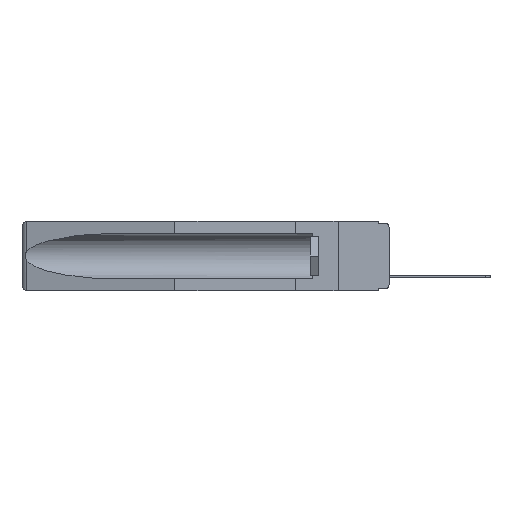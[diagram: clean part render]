
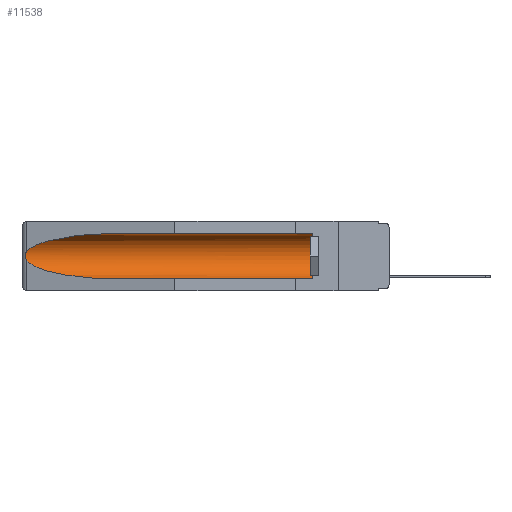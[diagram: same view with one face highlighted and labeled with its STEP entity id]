
A CAD part, left-side view. The second image highlights one B-rep face of the part: STEP entity #11538.
In plain terms, the highlighted cylindrical face has radius 2.857 mm (diameter 5.715 mm), a partial arc.
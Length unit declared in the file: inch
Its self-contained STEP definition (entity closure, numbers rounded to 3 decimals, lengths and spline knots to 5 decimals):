
#32 = CARTESIAN_POINT ( 'NONE',  ( 0.26537, 1.52718, -0.14972 ) ) ;
#301 = VECTOR ( 'NONE', #18161, 39.37008 ) ;
#348 = CARTESIAN_POINT ( 'NONE',  ( 0.155, 0.126, -0.059 ) ) ;
#428 = CARTESIAN_POINT ( 'NONE',  ( 0.26597, 1.5296, -0.19026 ) ) ;
#475 = CARTESIAN_POINT ( 'NONE',  ( 0.26537, 1.52718, -0.14972 ) ) ;
#616 = DIRECTION ( 'NONE',  ( 0., 0., 1. ) ) ;
#726 = CARTESIAN_POINT ( 'NONE',  ( 0.26537, 1.52718, -0.14972 ) ) ;
#1093 = ORIENTED_EDGE ( 'NONE', *, *, #1783, .F. ) ;
#1783 = EDGE_CURVE ( 'NONE', #4860, #5877, #4984, .T. ) ;
#1796 = ORIENTED_EDGE ( 'NONE', *, *, #17693, .T. ) ;
#2047 = CARTESIAN_POINT ( 'NONE',  ( 0.155, -0.30754, -0.1715 ) ) ;
#2898 = EDGE_CURVE ( 'NONE', #9815, #5777, #5706, .T. ) ;
#2907 = CIRCLE ( 'NONE', #16895, 0.1125 ) ;
#3389 = CARTESIAN_POINT ( 'NONE',  ( 0.155, -0.30754, -0.284 ) ) ;
#4310 = CARTESIAN_POINT ( 'NONE',  ( 0.155, 0.126, -0.1715 ) ) ;
#4643 = CARTESIAN_POINT ( 'NONE',  ( 0.155, 1.07973, -0.059 ) ) ;
#4745 = EDGE_CURVE ( 'NONE', #4860, #9815, #2907, .T. ) ;
#4860 = VERTEX_POINT ( 'NONE', #18361 ) ;
#4984 = LINE ( 'NONE', #3389, #15197 ) ;
#5153 = CARTESIAN_POINT ( 'NONE',  ( 0.26654, 1.53092, -0.15636 ) ) ;
#5706 = LINE ( 'NONE', #6013, #301 ) ;
#5777 = VERTEX_POINT ( 'NONE', #4643 ) ;
#5795 = CARTESIAN_POINT ( 'NONE',  ( 0.21114, 1.30732, -0.059 ) ) ;
#5877 = VERTEX_POINT ( 'NONE', #17292 ) ;
#6013 = CARTESIAN_POINT ( 'NONE',  ( 0.155, -0.30754, -0.059 ) ) ;
#7062 = ORIENTED_EDGE ( 'NONE', *, *, #11481, .T. ) ;
#7575 = CARTESIAN_POINT ( 'NONE',  ( 0.26537, 1.52718, -0.19328 ) ) ;
#8365 = CARTESIAN_POINT ( 'NONE',  ( 0.26537, 1.52718, -0.19328 ) ) ;
#8961 = CARTESIAN_POINT ( 'NONE',  ( 0.155, 1.07973, -0.059 ) ) ;
#9081 =( BOUNDED_CURVE ( )  B_SPLINE_CURVE ( 3, ( #8365, #18615, #19285, #9327 ),
 .UNSPECIFIED., .F., .F. ) 
 B_SPLINE_CURVE_WITH_KNOTS ( ( 4, 4 ),
 ( 0.1948, 1.5708 ),
 .UNSPECIFIED. ) 
 CURVE ( )  GEOMETRIC_REPRESENTATION_ITEM ( )  RATIONAL_B_SPLINE_CURVE ( ( 1., 0.848, 0.848, 1. ) ) 
 REPRESENTATION_ITEM ( '' )  );
#9327 = CARTESIAN_POINT ( 'NONE',  ( 0.155, 1.07973, -0.284 ) ) ;
#9484 = B_SPLINE_CURVE_WITH_KNOTS ( 'NONE', 3,
 ( #726, #15865, #5153, #15774, #17512, #11380, #17324, #14518, #428, #17715 ),
 .UNSPECIFIED., .F., .F.,
 ( 4, 2, 2, 2, 4 ),
 ( 0., 0.00029, 0.00058, 0.00087, 0.00117 ),
 .UNSPECIFIED. ) ;
#9815 = VERTEX_POINT ( 'NONE', #348 ) ;
#11107 = DIRECTION ( 'NONE',  ( 0., 1., 0. ) ) ;
#11277 = CYLINDRICAL_SURFACE ( 'NONE', #17722, 0.1125 ) ;
#11380 = CARTESIAN_POINT ( 'NONE',  ( 0.2675, 1.53308, -0.17534 ) ) ;
#11481 = EDGE_CURVE ( 'NONE', #14767, #13280, #9484, .T. ) ;
#11497 = ORIENTED_EDGE ( 'NONE', *, *, #16093, .T. ) ;
#11538 = ADVANCED_FACE ( 'NONE', ( #17418 ), #11277, .F. ) ;
#11799 = ORIENTED_EDGE ( 'NONE', *, *, #2898, .T. ) ;
#13139 = EDGE_LOOP ( 'NONE', ( #1796, #7062, #11497, #1093, #18824, #11799 ) ) ;
#13280 = VERTEX_POINT ( 'NONE', #7575 ) ;
#14518 = CARTESIAN_POINT ( 'NONE',  ( 0.26655, 1.53094, -0.18657 ) ) ;
#14767 = VERTEX_POINT ( 'NONE', #475 ) ;
#15197 = VECTOR ( 'NONE', #11107, 39.37008 ) ;
#15567 = CARTESIAN_POINT ( 'NONE',  ( 0.25451, 1.48313, -0.09465 ) ) ;
#15774 = CARTESIAN_POINT ( 'NONE',  ( 0.2673, 1.5327, -0.16383 ) ) ;
#15865 = CARTESIAN_POINT ( 'NONE',  ( 0.26597, 1.52961, -0.15275 ) ) ;
#16093 = EDGE_CURVE ( 'NONE', #13280, #5877, #9081, .T. ) ;
#16895 = AXIS2_PLACEMENT_3D ( 'NONE', #4310, #19882, #19577 ) ;
#17292 = CARTESIAN_POINT ( 'NONE',  ( 0.155, 1.07973, -0.284 ) ) ;
#17324 = CARTESIAN_POINT ( 'NONE',  ( 0.2673, 1.53269, -0.17917 ) ) ;
#17418 = FACE_OUTER_BOUND ( 'NONE', #13139, .T. ) ;
#17512 = CARTESIAN_POINT ( 'NONE',  ( 0.2675, 1.53308, -0.16763 ) ) ;
#17693 = EDGE_CURVE ( 'NONE', #5777, #14767, #18320, .T. ) ;
#17715 = CARTESIAN_POINT ( 'NONE',  ( 0.26537, 1.52718, -0.19328 ) ) ;
#17722 = AXIS2_PLACEMENT_3D ( 'NONE', #2047, #19032, #616 ) ;
#18161 = DIRECTION ( 'NONE',  ( 0., 1., 0. ) ) ;
#18320 =( BOUNDED_CURVE ( )  B_SPLINE_CURVE ( 3, ( #8961, #5795, #15567, #32 ),
 .UNSPECIFIED., .F., .F. ) 
 B_SPLINE_CURVE_WITH_KNOTS ( ( 4, 4 ),
 ( 4.71239, 6.08839 ),
 .UNSPECIFIED. ) 
 CURVE ( )  GEOMETRIC_REPRESENTATION_ITEM ( )  RATIONAL_B_SPLINE_CURVE ( ( 1., 0.848, 0.848, 1. ) ) 
 REPRESENTATION_ITEM ( '' )  );
#18361 = CARTESIAN_POINT ( 'NONE',  ( 0.155, 0.126, -0.284 ) ) ;
#18615 = CARTESIAN_POINT ( 'NONE',  ( 0.25451, 1.48313, -0.24835 ) ) ;
#18824 = ORIENTED_EDGE ( 'NONE', *, *, #4745, .T. ) ;
#19032 = DIRECTION ( 'NONE',  ( 0., 1., 0. ) ) ;
#19285 = CARTESIAN_POINT ( 'NONE',  ( 0.21114, 1.30732, -0.284 ) ) ;
#19577 = DIRECTION ( 'NONE',  ( 0., 0., 1. ) ) ;
#19882 = DIRECTION ( 'NONE',  ( 0., -1., 0. ) ) ;
